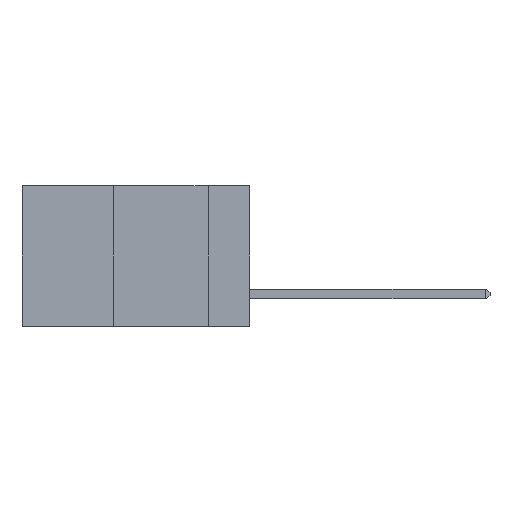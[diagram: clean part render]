
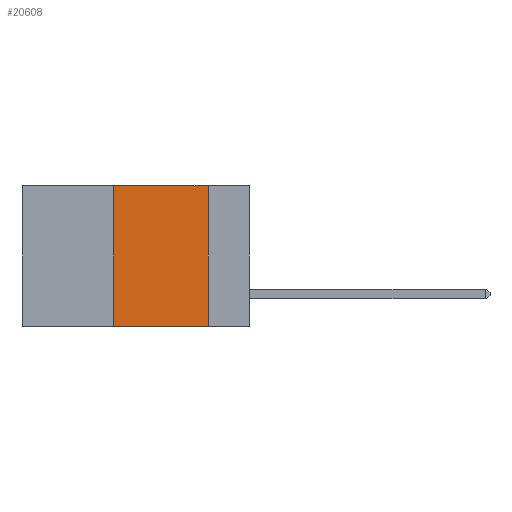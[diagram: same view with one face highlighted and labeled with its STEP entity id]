
A CAD part, left-side view. The second image highlights one B-rep face of the part: STEP entity #20608.
In plain terms, the highlighted planar face has unit normal (-1, 0, 0).
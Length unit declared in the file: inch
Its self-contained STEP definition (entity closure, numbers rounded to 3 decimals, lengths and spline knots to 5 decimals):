
#775 = EDGE_CURVE ( 'NONE', #13488, #10719, #16639, .T. ) ;
#2668 = ORIENTED_EDGE ( 'NONE', *, *, #8336, .F. ) ;
#4829 = PLANE ( 'NONE',  #5792 ) ;
#5792 = AXIS2_PLACEMENT_3D ( 'NONE', #14737, #27213, #12367 ) ;
#6705 = CARTESIAN_POINT ( 'NONE',  ( 0., 0.36, 0. ) ) ;
#6770 = LINE ( 'NONE', #9027, #25774 ) ;
#6779 = EDGE_LOOP ( 'NONE', ( #26081, #7872, #2668, #9420 ) ) ;
#7872 = ORIENTED_EDGE ( 'NONE', *, *, #775, .F. ) ;
#8336 = EDGE_CURVE ( 'NONE', #17502, #13488, #17708, .T. ) ;
#9027 = CARTESIAN_POINT ( 'NONE',  ( 0., 0.11, 0. ) ) ;
#9420 = ORIENTED_EDGE ( 'NONE', *, *, #10607, .T. ) ;
#10607 = EDGE_CURVE ( 'NONE', #17502, #18805, #17521, .T. ) ;
#10719 = VERTEX_POINT ( 'NONE', #25460 ) ;
#11298 = DIRECTION ( 'NONE',  ( 0., 0., 1. ) ) ;
#11497 = DIRECTION ( 'NONE',  ( 0., 0., -1. ) ) ;
#12367 = DIRECTION ( 'NONE',  ( 0., 0., -1. ) ) ;
#13488 = VERTEX_POINT ( 'NONE', #6705 ) ;
#14737 = CARTESIAN_POINT ( 'NONE',  ( 0., 0.6, 0. ) ) ;
#16639 = LINE ( 'NONE', #22220, #29050 ) ;
#16756 = VECTOR ( 'NONE', #29981, 39.37008 ) ;
#16942 = VECTOR ( 'NONE', #11298, 39.37008 ) ;
#17244 = EDGE_CURVE ( 'NONE', #10719, #18805, #6770, .T. ) ;
#17502 = VERTEX_POINT ( 'NONE', #24897 ) ;
#17521 = LINE ( 'NONE', #27528, #16756 ) ;
#17708 = LINE ( 'NONE', #18649, #16942 ) ;
#18649 = CARTESIAN_POINT ( 'NONE',  ( 0., 0.36, 0. ) ) ;
#18805 = VERTEX_POINT ( 'NONE', #27772 ) ;
#20608 = ADVANCED_FACE ( 'NONE', ( #24512 ), #4829, .F. ) ;
#22220 = CARTESIAN_POINT ( 'NONE',  ( 0., 0.6, 0. ) ) ;
#24512 = FACE_OUTER_BOUND ( 'NONE', #6779, .T. ) ;
#24681 = DIRECTION ( 'NONE',  ( 0., -1., 0. ) ) ;
#24897 = CARTESIAN_POINT ( 'NONE',  ( 0., 0.36, -0.37 ) ) ;
#25460 = CARTESIAN_POINT ( 'NONE',  ( 0., 0.11, 0. ) ) ;
#25774 = VECTOR ( 'NONE', #11497, 39.37008 ) ;
#26081 = ORIENTED_EDGE ( 'NONE', *, *, #17244, .F. ) ;
#27213 = DIRECTION ( 'NONE',  ( 1., 0., 0. ) ) ;
#27528 = CARTESIAN_POINT ( 'NONE',  ( 0., 0.6, -0.37 ) ) ;
#27772 = CARTESIAN_POINT ( 'NONE',  ( 0., 0.11, -0.37 ) ) ;
#29050 = VECTOR ( 'NONE', #24681, 39.37008 ) ;
#29981 = DIRECTION ( 'NONE',  ( 0., -1., 0. ) ) ;
